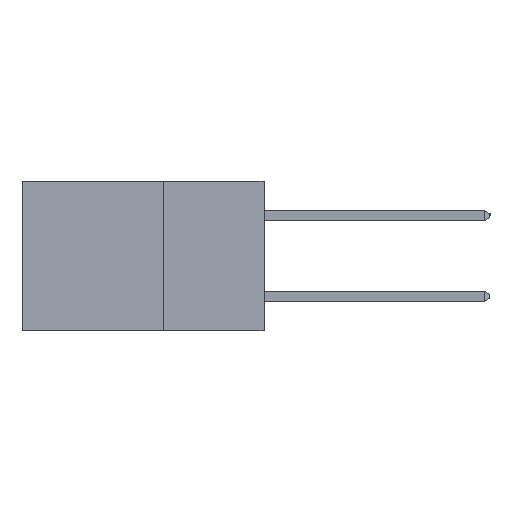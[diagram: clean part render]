
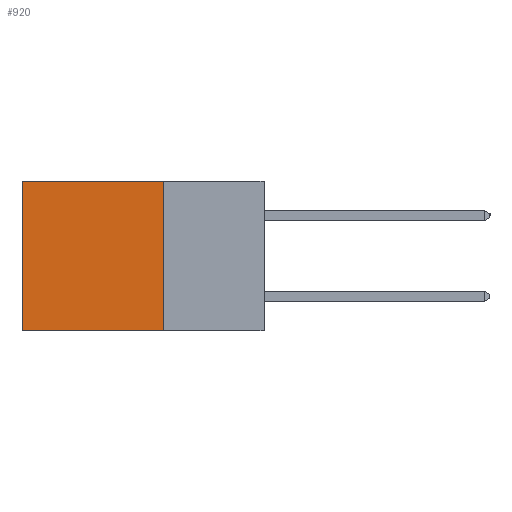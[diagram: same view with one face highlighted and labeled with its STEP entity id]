
A CAD part, left-side view. The second image highlights one B-rep face of the part: STEP entity #920.
In plain terms, the highlighted planar face has unit normal (-1, 0, 0).
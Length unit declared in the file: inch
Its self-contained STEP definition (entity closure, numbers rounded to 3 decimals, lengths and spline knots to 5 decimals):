
#255 = DIRECTION ( 'NONE',  ( 0., 1., 0. ) ) ;
#588 = ORIENTED_EDGE ( 'NONE', *, *, #1652, .F. ) ;
#920 = ADVANCED_FACE ( 'NONE', ( #9102 ), #2648, .F. ) ;
#1392 = CARTESIAN_POINT ( 'NONE',  ( 0.2615, 0.6, -0.37 ) ) ;
#1652 = EDGE_CURVE ( 'NONE', #13679, #3850, #11236, .T. ) ;
#1810 = VECTOR ( 'NONE', #2247, 39.37008 ) ;
#2247 = DIRECTION ( 'NONE',  ( 0., 0., -1. ) ) ;
#2277 = LINE ( 'NONE', #10103, #5899 ) ;
#2648 = PLANE ( 'NONE',  #10837 ) ;
#3850 = VERTEX_POINT ( 'NONE', #13284 ) ;
#4212 = ORIENTED_EDGE ( 'NONE', *, *, #4318, .T. ) ;
#4318 = EDGE_CURVE ( 'NONE', #13679, #4437, #2277, .T. ) ;
#4437 = VERTEX_POINT ( 'NONE', #11118 ) ;
#5211 = ORIENTED_EDGE ( 'NONE', *, *, #8674, .F. ) ;
#5262 = VECTOR ( 'NONE', #12398, 39.37008 ) ;
#5315 = EDGE_LOOP ( 'NONE', ( #11702, #5211, #588, #4212 ) ) ;
#5720 = VECTOR ( 'NONE', #9570, 39.37008 ) ;
#5774 = CARTESIAN_POINT ( 'NONE',  ( 0.2615, 0.25, -0.37 ) ) ;
#5899 = VECTOR ( 'NONE', #255, 39.37008 ) ;
#6237 = CARTESIAN_POINT ( 'NONE',  ( 0.2615, 0.6, -0.37 ) ) ;
#6509 = EDGE_CURVE ( 'NONE', #4437, #10530, #10890, .T. ) ;
#7484 = LINE ( 'NONE', #9854, #5720 ) ;
#7780 = CARTESIAN_POINT ( 'NONE',  ( 0.2615, 0.25, 0. ) ) ;
#7895 = DIRECTION ( 'NONE',  ( 0., 0., -1. ) ) ;
#7956 = CARTESIAN_POINT ( 'NONE',  ( 0.2615, 0.25, -0.37 ) ) ;
#8674 = EDGE_CURVE ( 'NONE', #3850, #10530, #7484, .T. ) ;
#9102 = FACE_OUTER_BOUND ( 'NONE', #5315, .T. ) ;
#9570 = DIRECTION ( 'NONE',  ( 0., 1., 0. ) ) ;
#9854 = CARTESIAN_POINT ( 'NONE',  ( 0.2615, 0.25, -0.37 ) ) ;
#10103 = CARTESIAN_POINT ( 'NONE',  ( 0.2615, 0.25, 0. ) ) ;
#10530 = VERTEX_POINT ( 'NONE', #6237 ) ;
#10837 = AXIS2_PLACEMENT_3D ( 'NONE', #7956, #11408, #7895 ) ;
#10890 = LINE ( 'NONE', #1392, #5262 ) ;
#11118 = CARTESIAN_POINT ( 'NONE',  ( 0.2615, 0.6, 0. ) ) ;
#11236 = LINE ( 'NONE', #5774, #1810 ) ;
#11408 = DIRECTION ( 'NONE',  ( 1., 0., 0. ) ) ;
#11702 = ORIENTED_EDGE ( 'NONE', *, *, #6509, .T. ) ;
#12398 = DIRECTION ( 'NONE',  ( 0., 0., -1. ) ) ;
#13284 = CARTESIAN_POINT ( 'NONE',  ( 0.2615, 0.25, -0.37 ) ) ;
#13679 = VERTEX_POINT ( 'NONE', #7780 ) ;
